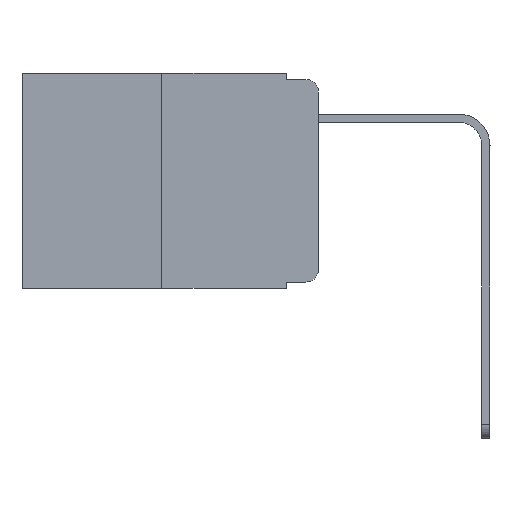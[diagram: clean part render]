
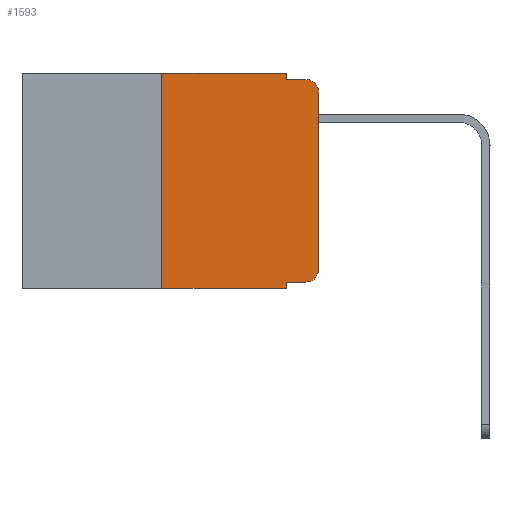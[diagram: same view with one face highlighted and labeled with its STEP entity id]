
A CAD part, left-side view. The second image highlights one B-rep face of the part: STEP entity #1593.
In plain terms, the highlighted planar face has unit normal (-1, 0, 0).
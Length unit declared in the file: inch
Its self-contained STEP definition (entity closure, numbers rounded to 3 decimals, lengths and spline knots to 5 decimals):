
#533 = DIRECTION ( 'NONE',  ( 0., 0., 1. ) ) ;
#633 = DIRECTION ( 'NONE',  ( 0., 0., -1. ) ) ;
#845 = EDGE_CURVE ( 'NONE', #10241, #12104, #6255, .T. ) ;
#977 = EDGE_CURVE ( 'NONE', #10241, #2964, #9794, .T. ) ;
#1137 = VECTOR ( 'NONE', #4068, 39.37008 ) ;
#1169 = EDGE_CURVE ( 'NONE', #2964, #5076, #12773, .T. ) ;
#1215 = ORIENTED_EDGE ( 'NONE', *, *, #6366, .T. ) ;
#1261 = VECTOR ( 'NONE', #1935, 39.37008 ) ;
#1460 = CARTESIAN_POINT ( 'NONE',  ( 0., 0.051, -0.343 ) ) ;
#1489 = DIRECTION ( 'NONE',  ( -1., 0., 0. ) ) ;
#1593 = ADVANCED_FACE ( 'NONE', ( #3135 ), #5884, .F. ) ;
#1631 = VECTOR ( 'NONE', #3951, 39.37008 ) ;
#1655 = CARTESIAN_POINT ( 'NONE',  ( 0., 0.051, -0.333 ) ) ;
#1734 = VECTOR ( 'NONE', #6427, 39.37008 ) ;
#1793 = EDGE_CURVE ( 'NONE', #8314, #8310, #11972, .T. ) ;
#1935 = DIRECTION ( 'NONE',  ( 0., -1., 0. ) ) ;
#2116 = CARTESIAN_POINT ( 'NONE',  ( 0., 0., 0. ) ) ;
#2373 = EDGE_CURVE ( 'NONE', #6345, #2709, #6760, .T. ) ;
#2709 = VERTEX_POINT ( 'NONE', #4464 ) ;
#2964 = VERTEX_POINT ( 'NONE', #6680 ) ;
#3135 = FACE_OUTER_BOUND ( 'NONE', #5087, .T. ) ;
#3265 = VECTOR ( 'NONE', #11048, 39.37008 ) ;
#3302 = CARTESIAN_POINT ( 'NONE',  ( 0., 0.25, 0. ) ) ;
#3336 = VERTEX_POINT ( 'NONE', #4149 ) ;
#3942 = CIRCLE ( 'NONE', #12800, 0.02 ) ;
#3951 = DIRECTION ( 'NONE',  ( 0., -1., 0. ) ) ;
#4068 = DIRECTION ( 'NONE',  ( 0., 0., 1. ) ) ;
#4149 = CARTESIAN_POINT ( 'NONE',  ( 0., 0., -0.03 ) ) ;
#4288 = ORIENTED_EDGE ( 'NONE', *, *, #977, .T. ) ;
#4301 = CARTESIAN_POINT ( 'NONE',  ( 0., 0.25, -0.343 ) ) ;
#4350 = ORIENTED_EDGE ( 'NONE', *, *, #2373, .F. ) ;
#4435 = EDGE_CURVE ( 'NONE', #2709, #7989, #12827, .T. ) ;
#4452 = LINE ( 'NONE', #2116, #1137 ) ;
#4464 = CARTESIAN_POINT ( 'NONE',  ( 0., 0.051, -0.01 ) ) ;
#4884 = CARTESIAN_POINT ( 'NONE',  ( 0., 0.473, 0. ) ) ;
#4996 = ORIENTED_EDGE ( 'NONE', *, *, #1169, .T. ) ;
#5076 = VERTEX_POINT ( 'NONE', #10779 ) ;
#5087 = EDGE_LOOP ( 'NONE', ( #10792, #1215, #12659, #4350, #10951, #10717, #8878, #9961, #4288, #4996 ) ) ;
#5547 = CARTESIAN_POINT ( 'NONE',  ( 0., 0.25, 0. ) ) ;
#5702 = CARTESIAN_POINT ( 'NONE',  ( 0., 0.051, 0. ) ) ;
#5884 = PLANE ( 'NONE',  #6482 ) ;
#6065 = CARTESIAN_POINT ( 'NONE',  ( 0., 0.051, 0. ) ) ;
#6255 = LINE ( 'NONE', #6065, #3265 ) ;
#6345 = VERTEX_POINT ( 'NONE', #5702 ) ;
#6366 = EDGE_CURVE ( 'NONE', #3336, #7989, #3942, .T. ) ;
#6427 = DIRECTION ( 'NONE',  ( 0., -1., 0. ) ) ;
#6482 = AXIS2_PLACEMENT_3D ( 'NONE', #4884, #12948, #11948 ) ;
#6680 = CARTESIAN_POINT ( 'NONE',  ( 0., 0.02, -0.333 ) ) ;
#6760 = LINE ( 'NONE', #10656, #10679 ) ;
#6919 = DIRECTION ( 'NONE',  ( 0., -1., 0. ) ) ;
#7228 = VECTOR ( 'NONE', #6919, 39.37008 ) ;
#7395 = VECTOR ( 'NONE', #533, 39.37008 ) ;
#7585 = DIRECTION ( 'NONE',  ( 0., 0., -1. ) ) ;
#7664 = DIRECTION ( 'NONE',  ( 0., 0., -1. ) ) ;
#7718 = EDGE_CURVE ( 'NONE', #8310, #6345, #7906, .T. ) ;
#7750 = DIRECTION ( 'NONE',  ( -1., 0., 0. ) ) ;
#7906 = LINE ( 'NONE', #7996, #1261 ) ;
#7989 = VERTEX_POINT ( 'NONE', #11768 ) ;
#7996 = CARTESIAN_POINT ( 'NONE',  ( 0., 0.473, 0. ) ) ;
#8310 = VERTEX_POINT ( 'NONE', #3302 ) ;
#8314 = VERTEX_POINT ( 'NONE', #4301 ) ;
#8319 = LINE ( 'NONE', #13035, #7228 ) ;
#8878 = ORIENTED_EDGE ( 'NONE', *, *, #9864, .T. ) ;
#9688 = CARTESIAN_POINT ( 'NONE',  ( 0., 0.02, -0.313 ) ) ;
#9794 = LINE ( 'NONE', #12448, #1734 ) ;
#9864 = EDGE_CURVE ( 'NONE', #8314, #12104, #8319, .T. ) ;
#9961 = ORIENTED_EDGE ( 'NONE', *, *, #845, .F. ) ;
#10241 = VERTEX_POINT ( 'NONE', #1655 ) ;
#10656 = CARTESIAN_POINT ( 'NONE',  ( 0., 0.051, 0. ) ) ;
#10679 = VECTOR ( 'NONE', #7664, 39.37008 ) ;
#10717 = ORIENTED_EDGE ( 'NONE', *, *, #1793, .F. ) ;
#10779 = CARTESIAN_POINT ( 'NONE',  ( 0., 0., -0.313 ) ) ;
#10792 = ORIENTED_EDGE ( 'NONE', *, *, #12576, .T. ) ;
#10873 = AXIS2_PLACEMENT_3D ( 'NONE', #9688, #7750, #633 ) ;
#10951 = ORIENTED_EDGE ( 'NONE', *, *, #7718, .F. ) ;
#11048 = DIRECTION ( 'NONE',  ( 0., 0., -1. ) ) ;
#11628 = CARTESIAN_POINT ( 'NONE',  ( 0., 0.02, -0.03 ) ) ;
#11768 = CARTESIAN_POINT ( 'NONE',  ( 0., 0.02, -0.01 ) ) ;
#11948 = DIRECTION ( 'NONE',  ( 0., 0., -1. ) ) ;
#11972 = LINE ( 'NONE', #5547, #7395 ) ;
#12104 = VERTEX_POINT ( 'NONE', #1460 ) ;
#12448 = CARTESIAN_POINT ( 'NONE',  ( 0., 0.051, -0.333 ) ) ;
#12576 = EDGE_CURVE ( 'NONE', #5076, #3336, #4452, .T. ) ;
#12659 = ORIENTED_EDGE ( 'NONE', *, *, #4435, .F. ) ;
#12773 = CIRCLE ( 'NONE', #10873, 0.02 ) ;
#12800 = AXIS2_PLACEMENT_3D ( 'NONE', #11628, #1489, #7585 ) ;
#12827 = LINE ( 'NONE', #12976, #1631 ) ;
#12948 = DIRECTION ( 'NONE',  ( 1., 0., 0. ) ) ;
#12976 = CARTESIAN_POINT ( 'NONE',  ( 0., 0.051, -0.01 ) ) ;
#13035 = CARTESIAN_POINT ( 'NONE',  ( 0., 0.473, -0.343 ) ) ;
